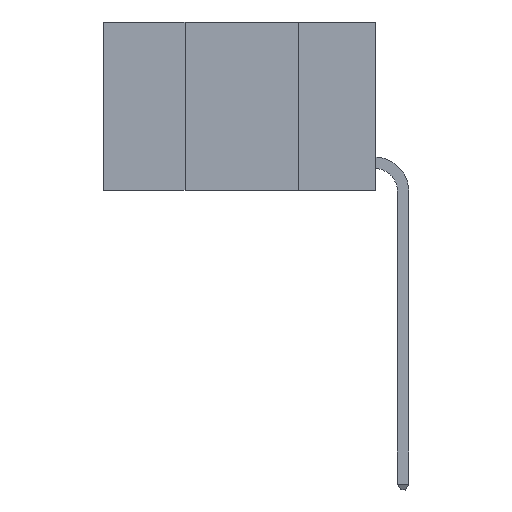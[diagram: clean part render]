
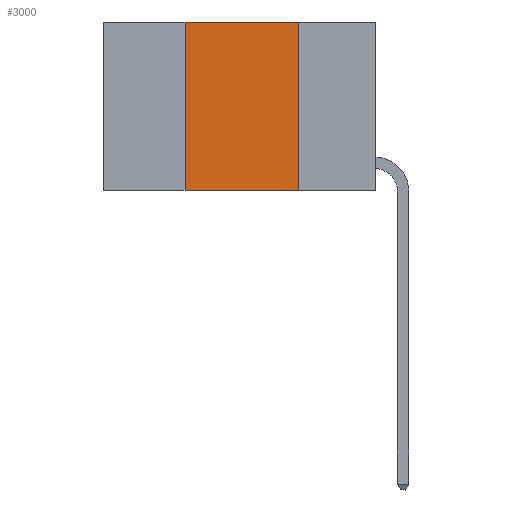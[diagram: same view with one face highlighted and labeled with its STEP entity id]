
A CAD part, left-side view. The second image highlights one B-rep face of the part: STEP entity #3000.
In plain terms, the highlighted planar face has unit normal (-1, 0, 0).
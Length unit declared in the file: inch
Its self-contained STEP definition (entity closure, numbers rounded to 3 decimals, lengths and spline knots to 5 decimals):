
#390 = VECTOR ( 'NONE', #15224, 39.37008 ) ;
#648 = PLANE ( 'NONE',  #4443 ) ;
#3000 = ADVANCED_FACE ( 'NONE', ( #3169 ), #648, .F. ) ;
#3163 = CARTESIAN_POINT ( 'NONE',  ( 0., 0.42, 0. ) ) ;
#3169 = FACE_OUTER_BOUND ( 'NONE', #21728, .T. ) ;
#3194 = ORIENTED_EDGE ( 'NONE', *, *, #12192, .F. ) ;
#3538 = DIRECTION ( 'NONE',  ( 0., 0., 1. ) ) ;
#4443 = AXIS2_PLACEMENT_3D ( 'NONE', #14782, #7781, #20137 ) ;
#4649 = LINE ( 'NONE', #14190, #8820 ) ;
#5039 = CARTESIAN_POINT ( 'NONE',  ( 0., 0.42, -0.37 ) ) ;
#5309 = ORIENTED_EDGE ( 'NONE', *, *, #14684, .T. ) ;
#6334 = CARTESIAN_POINT ( 'NONE',  ( 0., 0.17, 0. ) ) ;
#7074 = CARTESIAN_POINT ( 'NONE',  ( 0., 0.6, -0.37 ) ) ;
#7318 = VERTEX_POINT ( 'NONE', #5039 ) ;
#7781 = DIRECTION ( 'NONE',  ( 1., 0., 0. ) ) ;
#8188 = LINE ( 'NONE', #22012, #12375 ) ;
#8713 = VERTEX_POINT ( 'NONE', #9044 ) ;
#8820 = VECTOR ( 'NONE', #3538, 39.37008 ) ;
#8914 = CARTESIAN_POINT ( 'NONE',  ( 0., 0.17, 0. ) ) ;
#9044 = CARTESIAN_POINT ( 'NONE',  ( 0., 0.17, -0.37 ) ) ;
#12192 = EDGE_CURVE ( 'NONE', #7318, #20744, #4649, .T. ) ;
#12375 = VECTOR ( 'NONE', #13303, 39.37008 ) ;
#12467 = DIRECTION ( 'NONE',  ( 0., -1., 0. ) ) ;
#13303 = DIRECTION ( 'NONE',  ( 0., -1., 0. ) ) ;
#14190 = CARTESIAN_POINT ( 'NONE',  ( 0., 0.42, 0. ) ) ;
#14570 = LINE ( 'NONE', #6334, #390 ) ;
#14684 = EDGE_CURVE ( 'NONE', #7318, #8713, #15391, .T. ) ;
#14782 = CARTESIAN_POINT ( 'NONE',  ( 0., 0.6, 0. ) ) ;
#15224 = DIRECTION ( 'NONE',  ( 0., 0., -1. ) ) ;
#15391 = LINE ( 'NONE', #7074, #20046 ) ;
#16433 = VERTEX_POINT ( 'NONE', #8914 ) ;
#20046 = VECTOR ( 'NONE', #12467, 39.37008 ) ;
#20137 = DIRECTION ( 'NONE',  ( 0., 0., -1. ) ) ;
#20191 = ORIENTED_EDGE ( 'NONE', *, *, #21217, .F. ) ;
#20744 = VERTEX_POINT ( 'NONE', #3163 ) ;
#21217 = EDGE_CURVE ( 'NONE', #20744, #16433, #8188, .T. ) ;
#21564 = EDGE_CURVE ( 'NONE', #16433, #8713, #14570, .T. ) ;
#21728 = EDGE_LOOP ( 'NONE', ( #22617, #20191, #3194, #5309 ) ) ;
#22012 = CARTESIAN_POINT ( 'NONE',  ( 0., 0.6, 0. ) ) ;
#22617 = ORIENTED_EDGE ( 'NONE', *, *, #21564, .F. ) ;
